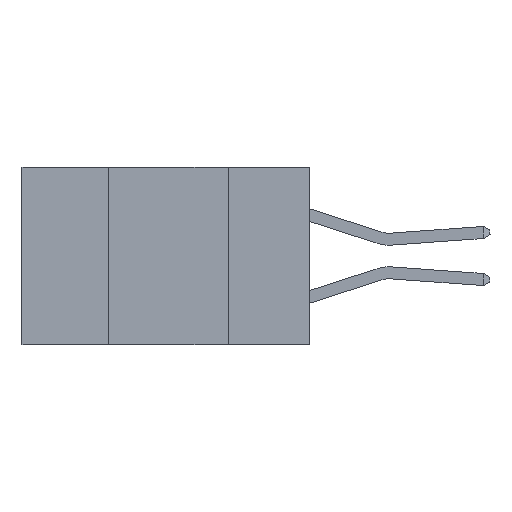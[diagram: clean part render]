
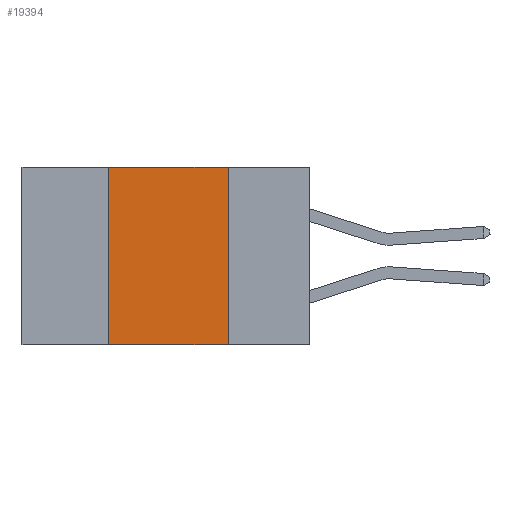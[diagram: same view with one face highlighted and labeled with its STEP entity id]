
A CAD part, left-side view. The second image highlights one B-rep face of the part: STEP entity #19394.
In plain terms, the highlighted planar face has unit normal (-1, 0, 0).
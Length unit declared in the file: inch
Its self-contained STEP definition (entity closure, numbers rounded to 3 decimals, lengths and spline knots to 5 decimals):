
#35 = CARTESIAN_POINT ( 'NONE',  ( 0., 0.17, -0.37 ) ) ;
#782 = AXIS2_PLACEMENT_3D ( 'NONE', #20994, #7907, #23209 ) ;
#1309 = PLANE ( 'NONE',  #782 ) ;
#1559 = CARTESIAN_POINT ( 'NONE',  ( 0., 0.6, 0. ) ) ;
#1856 = DIRECTION ( 'NONE',  ( 0., -1., 0. ) ) ;
#2252 = LINE ( 'NONE', #24926, #19000 ) ;
#3404 = FACE_OUTER_BOUND ( 'NONE', #7620, .T. ) ;
#5705 = LINE ( 'NONE', #28015, #22450 ) ;
#7611 = EDGE_CURVE ( 'NONE', #15320, #17786, #2252, .T. ) ;
#7620 = EDGE_LOOP ( 'NONE', ( #19973, #9766, #21349, #27148 ) ) ;
#7907 = DIRECTION ( 'NONE',  ( 1., 0., 0. ) ) ;
#9082 = DIRECTION ( 'NONE',  ( 0., 0., 1. ) ) ;
#9301 = VERTEX_POINT ( 'NONE', #11431 ) ;
#9766 = ORIENTED_EDGE ( 'NONE', *, *, #27149, .F. ) ;
#10365 = CARTESIAN_POINT ( 'NONE',  ( 0., 0.17, 0. ) ) ;
#11431 = CARTESIAN_POINT ( 'NONE',  ( 0., 0.42, 0. ) ) ;
#14895 = EDGE_CURVE ( 'NONE', #20555, #9301, #20585, .T. ) ;
#15320 = VERTEX_POINT ( 'NONE', #10365 ) ;
#17103 = VECTOR ( 'NONE', #18943, 39.37008 ) ;
#17457 = DIRECTION ( 'NONE',  ( 0., 0., -1. ) ) ;
#17786 = VERTEX_POINT ( 'NONE', #35 ) ;
#18943 = DIRECTION ( 'NONE',  ( 0., -1., 0. ) ) ;
#19000 = VECTOR ( 'NONE', #17457, 39.37008 ) ;
#19394 = ADVANCED_FACE ( 'NONE', ( #3404 ), #1309, .F. ) ;
#19973 = ORIENTED_EDGE ( 'NONE', *, *, #7611, .F. ) ;
#20555 = VERTEX_POINT ( 'NONE', #20625 ) ;
#20585 = LINE ( 'NONE', #26534, #25011 ) ;
#20625 = CARTESIAN_POINT ( 'NONE',  ( 0., 0.42, -0.37 ) ) ;
#20813 = EDGE_CURVE ( 'NONE', #20555, #17786, #5705, .T. ) ;
#20994 = CARTESIAN_POINT ( 'NONE',  ( 0., 0.6, 0. ) ) ;
#21349 = ORIENTED_EDGE ( 'NONE', *, *, #14895, .F. ) ;
#22450 = VECTOR ( 'NONE', #1856, 39.37008 ) ;
#22932 = LINE ( 'NONE', #1559, #17103 ) ;
#23209 = DIRECTION ( 'NONE',  ( 0., 0., -1. ) ) ;
#24926 = CARTESIAN_POINT ( 'NONE',  ( 0., 0.17, 0. ) ) ;
#25011 = VECTOR ( 'NONE', #9082, 39.37008 ) ;
#26534 = CARTESIAN_POINT ( 'NONE',  ( 0., 0.42, 0. ) ) ;
#27148 = ORIENTED_EDGE ( 'NONE', *, *, #20813, .T. ) ;
#27149 = EDGE_CURVE ( 'NONE', #9301, #15320, #22932, .T. ) ;
#28015 = CARTESIAN_POINT ( 'NONE',  ( 0., 0.6, -0.37 ) ) ;
